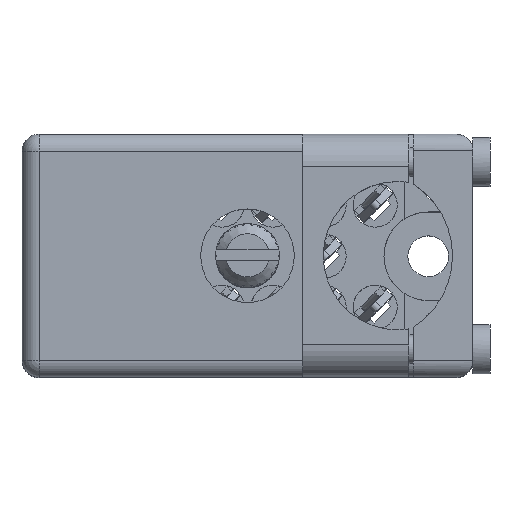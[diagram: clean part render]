
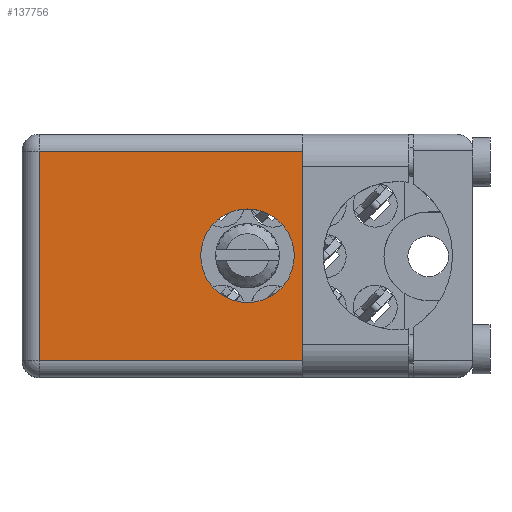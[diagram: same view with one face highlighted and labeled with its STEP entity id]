
A CAD part, top view. The second image highlights one B-rep face of the part: STEP entity #137756.
In plain terms, the highlighted face is planar.
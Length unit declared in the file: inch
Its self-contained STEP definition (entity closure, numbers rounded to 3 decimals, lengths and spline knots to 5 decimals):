
#1225 = AXIS2_PLACEMENT_3D ( 'NONE', #54715, #155147, #112587 ) ;
#1902 = CARTESIAN_POINT ( 'NONE',  ( 1.15, 0.906, -0.715 ) ) ;
#2066 = ORIENTED_EDGE ( 'NONE', *, *, #114873, .T. ) ;
#7963 = VERTEX_POINT ( 'NONE', #106982 ) ;
#10145 = EDGE_LOOP ( 'NONE', ( #52837, #119001, #27868, #2066, #16883, #44140, #51650, #42372 ) ) ;
#10148 = DIRECTION ( 'NONE',  ( 1., 0., 0. ) ) ;
#10237 = VERTEX_POINT ( 'NONE', #20408 ) ;
#10956 = CARTESIAN_POINT ( 'NONE',  ( 0.05, 0.906, -0.715 ) ) ;
#12705 = CARTESIAN_POINT ( 'NONE',  ( 0.865, 0.906, -0.6025 ) ) ;
#12873 = VERTEX_POINT ( 'NONE', #151034 ) ;
#16323 = DIRECTION ( 'NONE',  ( 0., 0., 1. ) ) ;
#16883 = ORIENTED_EDGE ( 'NONE', *, *, #98227, .T. ) ;
#20267 = EDGE_LOOP ( 'NONE', ( #152329, #156137 ) ) ;
#20408 = CARTESIAN_POINT ( 'NONE',  ( 0.05, 0.906, -0.05 ) ) ;
#21510 = CARTESIAN_POINT ( 'NONE',  ( 0.6625, 0.906, -0.495 ) ) ;
#23145 = VERTEX_POINT ( 'NONE', #32127 ) ;
#23984 = CARTESIAN_POINT ( 'NONE',  ( 1.15, 0.906, -0.05 ) ) ;
#27868 = ORIENTED_EDGE ( 'NONE', *, *, #48244, .F. ) ;
#30291 = CARTESIAN_POINT ( 'NONE',  ( 0.865, 0.906, -0.6025 ) ) ;
#32127 = CARTESIAN_POINT ( 'NONE',  ( 0.6625, 0.906, -0.22 ) ) ;
#32821 = VECTOR ( 'NONE', #152825, 39.37008 ) ;
#34744 = VERTEX_POINT ( 'NONE', #123373 ) ;
#34836 = PLANE ( 'NONE',  #182837 ) ;
#37754 = FACE_OUTER_BOUND ( 'NONE', #10145, .T. ) ;
#42363 = LINE ( 'NONE', #85468, #73807 ) ;
#42372 = ORIENTED_EDGE ( 'NONE', *, *, #125803, .T. ) ;
#43717 = DIRECTION ( 'NONE',  ( 0., 0., -1. ) ) ;
#44140 = ORIENTED_EDGE ( 'NONE', *, *, #86868, .T. ) ;
#48244 = EDGE_CURVE ( 'NONE', #69194, #34744, #79893, .T. ) ;
#49162 = CARTESIAN_POINT ( 'NONE',  ( 0., 0.906, -0.715 ) ) ;
#50948 = EDGE_CURVE ( 'NONE', #91122, #23145, #137485, .T. ) ;
#51218 = CARTESIAN_POINT ( 'NONE',  ( 0.865, 0.906, -0.1125 ) ) ;
#51650 = ORIENTED_EDGE ( 'NONE', *, *, #168757, .F. ) ;
#52837 = ORIENTED_EDGE ( 'NONE', *, *, #119253, .T. ) ;
#54227 = DIRECTION ( 'NONE',  ( -1., 0., 0. ) ) ;
#54715 = CARTESIAN_POINT ( 'NONE',  ( 0.6625, 0.906, -0.3575 ) ) ;
#55239 = VECTOR ( 'NONE', #111341, 39.37008 ) ;
#61170 = DIRECTION ( 'NONE',  ( 0., 1., 0. ) ) ;
#63797 = VERTEX_POINT ( 'NONE', #12705 ) ;
#67886 = VECTOR ( 'NONE', #43717, 39.37008 ) ;
#69194 = VERTEX_POINT ( 'NONE', #178267 ) ;
#73467 = DIRECTION ( 'NONE',  ( 1., 0., 0. ) ) ;
#73807 = VECTOR ( 'NONE', #172581, 39.37008 ) ;
#76861 = DIRECTION ( 'NONE',  ( 0., 0., 1. ) ) ;
#79893 = LINE ( 'NONE', #81927, #32821 ) ;
#80365 = FACE_BOUND ( 'NONE', #20267, .T. ) ;
#81927 = CARTESIAN_POINT ( 'NONE',  ( 1.15, 0.906, -0.715 ) ) ;
#82050 = LINE ( 'NONE', #30291, #180845 ) ;
#84959 = CIRCLE ( 'NONE', #120130, 0.1375 ) ;
#85468 = CARTESIAN_POINT ( 'NONE',  ( 0.865, 0.906, -0.1125 ) ) ;
#86868 = EDGE_CURVE ( 'NONE', #63797, #154687, #82050, .T. ) ;
#87377 = LINE ( 'NONE', #1902, #152503 ) ;
#91122 = VERTEX_POINT ( 'NONE', #21510 ) ;
#98056 = LINE ( 'NONE', #10956, #55239 ) ;
#98227 = EDGE_CURVE ( 'NONE', #12873, #63797, #139819, .T. ) ;
#106982 = CARTESIAN_POINT ( 'NONE',  ( 1.15, 0.906, -0.665 ) ) ;
#111341 = DIRECTION ( 'NONE',  ( 0., 0., 1. ) ) ;
#112587 = DIRECTION ( 'NONE',  ( 0., 0., 1. ) ) ;
#114858 = LINE ( 'NONE', #23984, #184345 ) ;
#114873 = EDGE_CURVE ( 'NONE', #69194, #12873, #42363, .T. ) ;
#118440 = CARTESIAN_POINT ( 'NONE',  ( 0.6625, 0.906, -0.3575 ) ) ;
#119001 = ORIENTED_EDGE ( 'NONE', *, *, #120741, .T. ) ;
#119253 = EDGE_CURVE ( 'NONE', #120300, #10237, #98056, .T. ) ;
#120130 = AXIS2_PLACEMENT_3D ( 'NONE', #118440, #61170, #76861 ) ;
#120300 = VERTEX_POINT ( 'NONE', #140587 ) ;
#120741 = EDGE_CURVE ( 'NONE', #10237, #34744, #114858, .T. ) ;
#120934 = CARTESIAN_POINT ( 'NONE',  ( 1.15, 0.906, -0.6025 ) ) ;
#123361 = VECTOR ( 'NONE', #54227, 39.37008 ) ;
#123373 = CARTESIAN_POINT ( 'NONE',  ( 1.15, 0.906, -0.05 ) ) ;
#125803 = EDGE_CURVE ( 'NONE', #7963, #120300, #143453, .T. ) ;
#126268 = EDGE_CURVE ( 'NONE', #23145, #91122, #84959, .T. ) ;
#137485 = CIRCLE ( 'NONE', #1225, 0.1375 ) ;
#137756 = ADVANCED_FACE ( 'NONE', ( #37754, #80365 ), #34836, .T. ) ;
#139819 = LINE ( 'NONE', #51218, #67886 ) ;
#140587 = CARTESIAN_POINT ( 'NONE',  ( 0.05, 0.906, -0.665 ) ) ;
#143453 = LINE ( 'NONE', #156523, #123361 ) ;
#151034 = CARTESIAN_POINT ( 'NONE',  ( 0.865, 0.906, -0.1125 ) ) ;
#152329 = ORIENTED_EDGE ( 'NONE', *, *, #126268, .F. ) ;
#152503 = VECTOR ( 'NONE', #16323, 39.37008 ) ;
#152825 = DIRECTION ( 'NONE',  ( 0., 0., 1. ) ) ;
#154687 = VERTEX_POINT ( 'NONE', #120934 ) ;
#155147 = DIRECTION ( 'NONE',  ( 0., 1., 0. ) ) ;
#156137 = ORIENTED_EDGE ( 'NONE', *, *, #50948, .F. ) ;
#156523 = CARTESIAN_POINT ( 'NONE',  ( 0., 0.906, -0.665 ) ) ;
#163953 = DIRECTION ( 'NONE',  ( 0., 1., 0. ) ) ;
#168757 = EDGE_CURVE ( 'NONE', #7963, #154687, #87377, .T. ) ;
#172581 = DIRECTION ( 'NONE',  ( -1., 0., 0. ) ) ;
#178267 = CARTESIAN_POINT ( 'NONE',  ( 1.15, 0.906, -0.1125 ) ) ;
#179615 = DIRECTION ( 'NONE',  ( 0., 0., 1. ) ) ;
#180845 = VECTOR ( 'NONE', #73467, 39.37008 ) ;
#182837 = AXIS2_PLACEMENT_3D ( 'NONE', #49162, #163953, #179615 ) ;
#184345 = VECTOR ( 'NONE', #10148, 39.37008 ) ;
